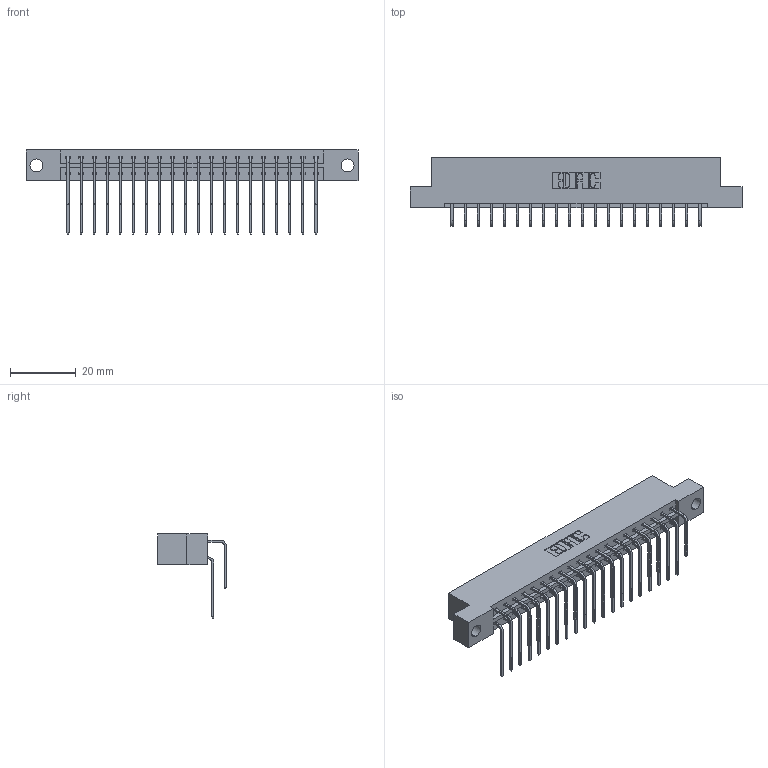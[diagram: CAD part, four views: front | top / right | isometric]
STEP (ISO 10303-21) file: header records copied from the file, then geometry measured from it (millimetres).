
FILE_DESCRIPTION (( 'STEP AP203' ), '1' );
FILE_NAME ('833-040-559-204.STEP', '2020-06-03T18:12:02', ( '' ), ( '' ), 'SwSTEP 2.0', 'SolidWorks 2020', '' );
FILE_SCHEMA (( 'CONFIG_CONTROL_DESIGN' ));
Length unit declared in the file: inch
Products named in the file (4): 345-292-001_558 559 Tail - 1; 833-040-559-204; 345-292-001_559 Tail - 2; 833 Part_Flush - .156 Dia - TH
Assembly tree (41 placements, depth 2):
  833-040-559-204
    833 Part_Flush - .156 Dia - TH
    345-292-001_558 559 Tail - 1  x20
    345-292-001_559 Tail - 2  x20
Bounding box: 100.79 x 20.9 x 25.53 mm (x, y, z)
Volume: 10227 mm3; surface area: 12803.2 mm2
Topology: 41 solids, 41 shells, 2274 faces, 6751 edges, 4446 vertices
Faces by surface type: plane 1590, cylinder 684
Entity records: 17499 total; most frequent: CARTESIAN_POINT 2977, ORIENTED_EDGE 2862, DIRECTION 2563, EDGE_CURVE 1431, VECTOR 1263, LINE 1263, VERTEX_POINT 950, AXIS2_PLACEMENT_3D 650
